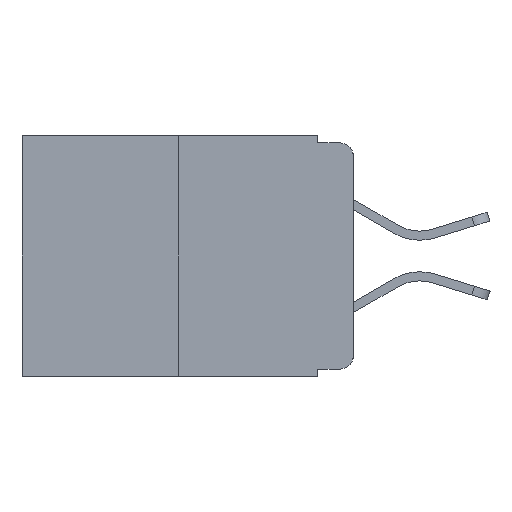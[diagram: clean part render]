
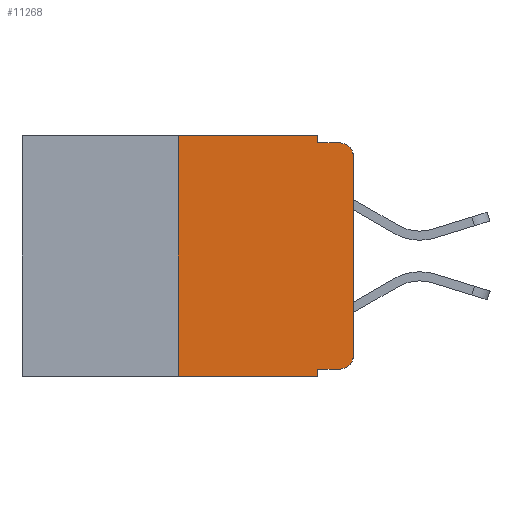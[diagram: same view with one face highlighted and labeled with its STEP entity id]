
A CAD part, left-side view. The second image highlights one B-rep face of the part: STEP entity #11268.
In plain terms, the highlighted planar face has unit normal (-1, 0, 0).
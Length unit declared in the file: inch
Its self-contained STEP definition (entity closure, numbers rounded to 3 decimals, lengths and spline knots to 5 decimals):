
#150 = DIRECTION ( 'NONE',  ( -1., 0., 0. ) ) ;
#154 = FACE_OUTER_BOUND ( 'NONE', #3240, .T. ) ;
#517 = AXIS2_PLACEMENT_3D ( 'NONE', #5986, #4971, #908 ) ;
#623 = DIRECTION ( 'NONE',  ( 0., -1., 0. ) ) ;
#715 = DIRECTION ( 'NONE',  ( 0., 0., -1. ) ) ;
#734 = VECTOR ( 'NONE', #1279, 39.37008 ) ;
#758 = ORIENTED_EDGE ( 'NONE', *, *, #7874, .T. ) ;
#778 = EDGE_CURVE ( 'NONE', #5290, #2764, #11530, .T. ) ;
#908 = DIRECTION ( 'NONE',  ( 0., 0., -1. ) ) ;
#1102 = CARTESIAN_POINT ( 'NONE',  ( 0., 0.25, 0. ) ) ;
#1103 = VERTEX_POINT ( 'NONE', #7853 ) ;
#1279 = DIRECTION ( 'NONE',  ( 0., 0., 1. ) ) ;
#2046 = ORIENTED_EDGE ( 'NONE', *, *, #9104, .F. ) ;
#2764 = VERTEX_POINT ( 'NONE', #13155 ) ;
#2904 = VERTEX_POINT ( 'NONE', #1102 ) ;
#3187 = DIRECTION ( 'NONE',  ( 0., 0., -1. ) ) ;
#3240 = EDGE_LOOP ( 'NONE', ( #5877, #8435, #3745, #3945, #2046, #8562, #11107, #11928, #9327, #758 ) ) ;
#3407 = VERTEX_POINT ( 'NONE', #12661 ) ;
#3445 = CARTESIAN_POINT ( 'NONE',  ( 0., 0., -0.03 ) ) ;
#3670 = EDGE_CURVE ( 'NONE', #7748, #5290, #9329, .T. ) ;
#3745 = ORIENTED_EDGE ( 'NONE', *, *, #11041, .F. ) ;
#3805 = VECTOR ( 'NONE', #715, 39.37008 ) ;
#3866 = VERTEX_POINT ( 'NONE', #10483 ) ;
#3911 = VECTOR ( 'NONE', #7761, 39.37008 ) ;
#3945 = ORIENTED_EDGE ( 'NONE', *, *, #6220, .F. ) ;
#4034 = CARTESIAN_POINT ( 'NONE',  ( 0., 0.473, 0. ) ) ;
#4566 = CARTESIAN_POINT ( 'NONE',  ( 0., 0.051, -0.333 ) ) ;
#4730 = LINE ( 'NONE', #13109, #3911 ) ;
#4840 = CARTESIAN_POINT ( 'NONE',  ( 0., 0.051, -0.343 ) ) ;
#4971 = DIRECTION ( 'NONE',  ( -1., 0., 0. ) ) ;
#5053 = LINE ( 'NONE', #5860, #3805 ) ;
#5225 = DIRECTION ( 'NONE',  ( 0., 0., -1. ) ) ;
#5290 = VERTEX_POINT ( 'NONE', #3445 ) ;
#5860 = CARTESIAN_POINT ( 'NONE',  ( 0., 0.051, 0. ) ) ;
#5877 = ORIENTED_EDGE ( 'NONE', *, *, #3670, .T. ) ;
#5986 = CARTESIAN_POINT ( 'NONE',  ( 0., 0.02, -0.313 ) ) ;
#6010 = DIRECTION ( 'NONE',  ( 0., -1., 0. ) ) ;
#6094 = AXIS2_PLACEMENT_3D ( 'NONE', #4034, #8149, #12265 ) ;
#6119 = AXIS2_PLACEMENT_3D ( 'NONE', #8471, #150, #5225 ) ;
#6220 = EDGE_CURVE ( 'NONE', #12437, #3407, #5053, .T. ) ;
#6364 = LINE ( 'NONE', #11571, #734 ) ;
#6955 = LINE ( 'NONE', #8315, #10012 ) ;
#6985 = VECTOR ( 'NONE', #11269, 39.37008 ) ;
#7141 = CARTESIAN_POINT ( 'NONE',  ( 0., 0.051, -0.333 ) ) ;
#7748 = VERTEX_POINT ( 'NONE', #12571 ) ;
#7761 = DIRECTION ( 'NONE',  ( 0., -1., 0. ) ) ;
#7853 = CARTESIAN_POINT ( 'NONE',  ( 0., 0.25, -0.343 ) ) ;
#7874 = EDGE_CURVE ( 'NONE', #3866, #7748, #9498, .T. ) ;
#8016 = VECTOR ( 'NONE', #10346, 39.37008 ) ;
#8108 = VERTEX_POINT ( 'NONE', #4566 ) ;
#8149 = DIRECTION ( 'NONE',  ( 1., 0., 0. ) ) ;
#8165 = LINE ( 'NONE', #7141, #6985 ) ;
#8315 = CARTESIAN_POINT ( 'NONE',  ( 0., 0.473, -0.343 ) ) ;
#8435 = ORIENTED_EDGE ( 'NONE', *, *, #778, .T. ) ;
#8471 = CARTESIAN_POINT ( 'NONE',  ( 0., 0.02, -0.03 ) ) ;
#8562 = ORIENTED_EDGE ( 'NONE', *, *, #12960, .F. ) ;
#9104 = EDGE_CURVE ( 'NONE', #2904, #12437, #4730, .T. ) ;
#9327 = ORIENTED_EDGE ( 'NONE', *, *, #12471, .T. ) ;
#9329 = LINE ( 'NONE', #9402, #8016 ) ;
#9402 = CARTESIAN_POINT ( 'NONE',  ( 0., 0., 0. ) ) ;
#9498 = CIRCLE ( 'NONE', #517, 0.02 ) ;
#9780 = VECTOR ( 'NONE', #623, 39.37008 ) ;
#10012 = VECTOR ( 'NONE', #6010, 39.37008 ) ;
#10084 = LINE ( 'NONE', #11534, #10680 ) ;
#10262 = CARTESIAN_POINT ( 'NONE',  ( 0., 0.051, 0. ) ) ;
#10346 = DIRECTION ( 'NONE',  ( 0., 0., 1. ) ) ;
#10483 = CARTESIAN_POINT ( 'NONE',  ( 0., 0.02, -0.333 ) ) ;
#10680 = VECTOR ( 'NONE', #3187, 39.37008 ) ;
#10842 = CARTESIAN_POINT ( 'NONE',  ( 0., 0.051, -0.01 ) ) ;
#10972 = LINE ( 'NONE', #10842, #9780 ) ;
#11041 = EDGE_CURVE ( 'NONE', #3407, #2764, #10972, .T. ) ;
#11107 = ORIENTED_EDGE ( 'NONE', *, *, #11907, .T. ) ;
#11268 = ADVANCED_FACE ( 'NONE', ( #154 ), #13295, .F. ) ;
#11269 = DIRECTION ( 'NONE',  ( 0., -1., 0. ) ) ;
#11530 = CIRCLE ( 'NONE', #6119, 0.02 ) ;
#11534 = CARTESIAN_POINT ( 'NONE',  ( 0., 0.051, 0. ) ) ;
#11571 = CARTESIAN_POINT ( 'NONE',  ( 0., 0.25, 0. ) ) ;
#11907 = EDGE_CURVE ( 'NONE', #1103, #12784, #6955, .T. ) ;
#11928 = ORIENTED_EDGE ( 'NONE', *, *, #13226, .F. ) ;
#12265 = DIRECTION ( 'NONE',  ( 0., 0., -1. ) ) ;
#12437 = VERTEX_POINT ( 'NONE', #10262 ) ;
#12471 = EDGE_CURVE ( 'NONE', #8108, #3866, #8165, .T. ) ;
#12571 = CARTESIAN_POINT ( 'NONE',  ( 0., 0., -0.313 ) ) ;
#12661 = CARTESIAN_POINT ( 'NONE',  ( 0., 0.051, -0.01 ) ) ;
#12784 = VERTEX_POINT ( 'NONE', #4840 ) ;
#12960 = EDGE_CURVE ( 'NONE', #1103, #2904, #6364, .T. ) ;
#13109 = CARTESIAN_POINT ( 'NONE',  ( 0., 0.473, 0. ) ) ;
#13155 = CARTESIAN_POINT ( 'NONE',  ( 0., 0.02, -0.01 ) ) ;
#13226 = EDGE_CURVE ( 'NONE', #8108, #12784, #10084, .T. ) ;
#13295 = PLANE ( 'NONE',  #6094 ) ;
